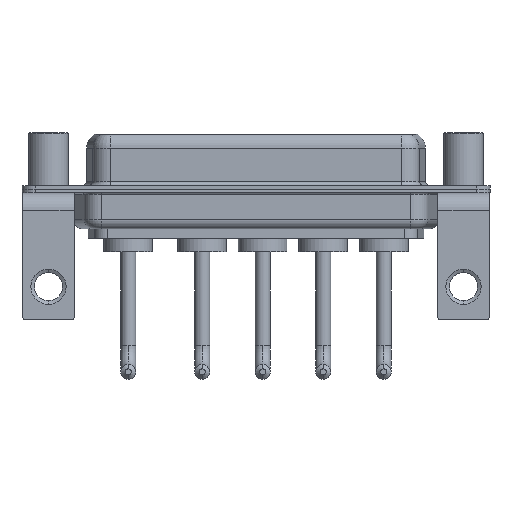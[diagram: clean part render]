
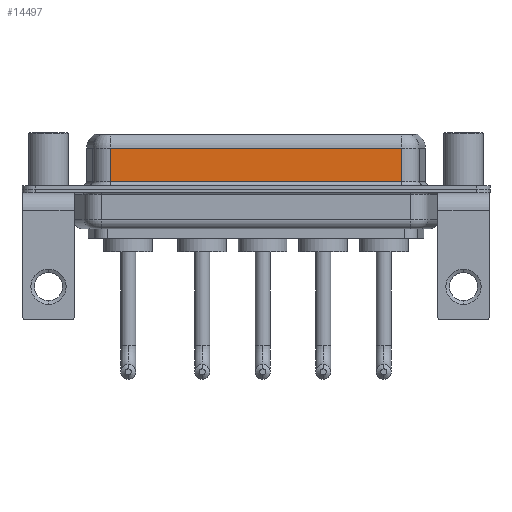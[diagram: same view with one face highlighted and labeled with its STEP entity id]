
A CAD part, front view. The second image highlights one B-rep face of the part: STEP entity #14497.
In plain terms, the highlighted planar face has unit normal (0, -1, 0).
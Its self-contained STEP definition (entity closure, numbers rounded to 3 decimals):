
#801 = VECTOR ( 'NONE', #4317, 1000. ) ;
#1683 = EDGE_CURVE ( 'NONE', #4692, #2372, #2546, .T. ) ;
#1840 = CARTESIAN_POINT ( 'NONE',  ( 40.037, -3.95, 6.4 ) ) ;
#1920 = ORIENTED_EDGE ( 'NONE', *, *, #11279, .T. ) ;
#2179 = ORIENTED_EDGE ( 'NONE', *, *, #6521, .F. ) ;
#2269 = VECTOR ( 'NONE', #5647, 1000. ) ;
#2372 = VERTEX_POINT ( 'NONE', #9725 ) ;
#2546 = LINE ( 'NONE', #4783, #10048 ) ;
#2563 = CARTESIAN_POINT ( 'NONE',  ( 40.037, -3.95, 4.65 ) ) ;
#2975 = FACE_OUTER_BOUND ( 'NONE', #12020, .T. ) ;
#4317 = DIRECTION ( 'NONE',  ( -1., 0., 0. ) ) ;
#4692 = VERTEX_POINT ( 'NONE', #14003 ) ;
#4716 = EDGE_CURVE ( 'NONE', #2372, #13436, #7034, .T. ) ;
#4783 = CARTESIAN_POINT ( 'NONE',  ( 7.013, -3.95, 6.4 ) ) ;
#4787 = DIRECTION ( 'NONE',  ( 0., 0., 1. ) ) ;
#5647 = DIRECTION ( 'NONE',  ( 1., 0., 0. ) ) ;
#6246 = LINE ( 'NONE', #11907, #8059 ) ;
#6521 = EDGE_CURVE ( 'NONE', #11069, #13436, #6246, .T. ) ;
#7034 = LINE ( 'NONE', #10209, #2269 ) ;
#7203 = ORIENTED_EDGE ( 'NONE', *, *, #4716, .T. ) ;
#7257 = DIRECTION ( 'NONE',  ( 0., 0., -1. ) ) ;
#7681 = PLANE ( 'NONE',  #12667 ) ;
#8059 = VECTOR ( 'NONE', #7257, 1000. ) ;
#9501 = DIRECTION ( 'NONE',  ( 0., 0., -1. ) ) ;
#9725 = CARTESIAN_POINT ( 'NONE',  ( 7.013, -3.95, 0.9 ) ) ;
#10048 = VECTOR ( 'NONE', #9501, 1000. ) ;
#10098 = ORIENTED_EDGE ( 'NONE', *, *, #1683, .T. ) ;
#10209 = CARTESIAN_POINT ( 'NONE',  ( 40.037, -3.95, 0.9 ) ) ;
#10665 = DIRECTION ( 'NONE',  ( 0., 1., 0. ) ) ;
#11069 = VERTEX_POINT ( 'NONE', #2563 ) ;
#11279 = EDGE_CURVE ( 'NONE', #11069, #4692, #11429, .T. ) ;
#11429 = LINE ( 'NONE', #13682, #801 ) ;
#11907 = CARTESIAN_POINT ( 'NONE',  ( 40.037, -3.95, 6.4 ) ) ;
#12020 = EDGE_LOOP ( 'NONE', ( #2179, #1920, #10098, #7203 ) ) ;
#12667 = AXIS2_PLACEMENT_3D ( 'NONE', #1840, #10665, #4787 ) ;
#13436 = VERTEX_POINT ( 'NONE', #15190 ) ;
#13682 = CARTESIAN_POINT ( 'NONE',  ( 40.037, -3.95, 4.65 ) ) ;
#14003 = CARTESIAN_POINT ( 'NONE',  ( 7.013, -3.95, 4.65 ) ) ;
#14497 = ADVANCED_FACE ( 'NONE', ( #2975 ), #7681, .F. ) ;
#15190 = CARTESIAN_POINT ( 'NONE',  ( 40.037, -3.95, 0.9 ) ) ;
